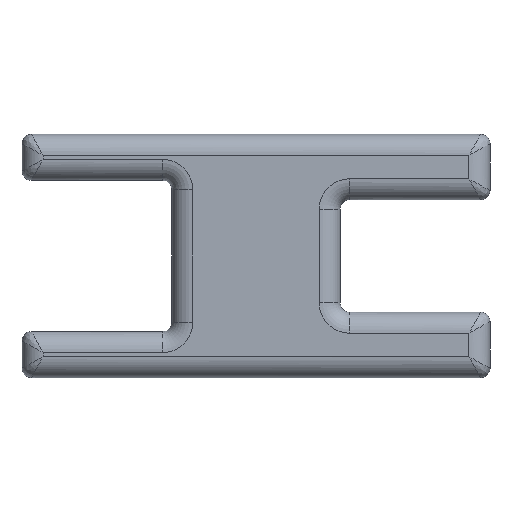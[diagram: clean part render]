
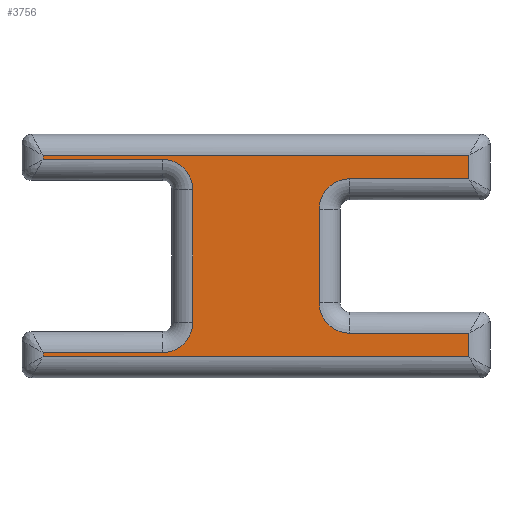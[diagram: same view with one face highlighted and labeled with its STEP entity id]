
A CAD part, front view. The second image highlights one B-rep face of the part: STEP entity #3756.
In plain terms, the highlighted planar face has unit normal (0, -1, 0).
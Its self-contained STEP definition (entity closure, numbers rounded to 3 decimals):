
#108=CIRCLE('',#3889,3.25);
#110=CIRCLE('',#3893,3.25);
#114=CIRCLE('',#3902,3.25);
#118=CIRCLE('',#3908,3.25);
#615=FACE_OUTER_BOUND('',#846,.T.);
#846=EDGE_LOOP('',(#3343,#3344,#3345,#3346,#3347,#3348,#3349,#3350,#3351,
#3352,#3353,#3354,#3355,#3356,#3357,#3358));
#1123=LINE('',#7339,#1422);
#1125=LINE('',#7348,#1424);
#1128=LINE('',#7360,#1427);
#1130=LINE('',#7366,#1429);
#1132=LINE('',#7369,#1431);
#1134=LINE('',#7372,#1433);
#1135=LINE('',#7375,#1434);
#1138=LINE('',#7390,#1437);
#1140=LINE('',#7399,#1439);
#1142=LINE('',#7402,#1441);
#1144=LINE('',#7405,#1443);
#1146=LINE('',#7408,#1445);
#1422=VECTOR('',#4404,10.);
#1424=VECTOR('',#4412,10.);
#1427=VECTOR('',#4427,10.);
#1429=VECTOR('',#4437,10.);
#1431=VECTOR('',#4441,10.);
#1433=VECTOR('',#4445,10.);
#1434=VECTOR('',#4448,10.);
#1437=VECTOR('',#4465,10.);
#1439=VECTOR('',#4477,10.);
#1441=VECTOR('',#4481,10.);
#1443=VECTOR('',#4485,10.);
#1445=VECTOR('',#4489,10.);
#1770=VERTEX_POINT('',#7082);
#1773=VERTEX_POINT('',#7118);
#1776=VERTEX_POINT('',#7154);
#1779=VERTEX_POINT('',#7190);
#1782=VERTEX_POINT('',#7226);
#1785=VERTEX_POINT('',#7262);
#1788=VERTEX_POINT('',#7298);
#1791=VERTEX_POINT('',#7334);
#1792=VERTEX_POINT('',#7338);
#1795=VERTEX_POINT('',#7345);
#1796=VERTEX_POINT('',#7347);
#1798=VERTEX_POINT('',#7353);
#1800=VERTEX_POINT('',#7374);
#1802=VERTEX_POINT('',#7380);
#1804=VERTEX_POINT('',#7386);
#1806=VERTEX_POINT('',#7392);
#2277=EDGE_CURVE('',#1770,#1792,#1123,.T.);
#2281=EDGE_CURVE('',#1795,#1796,#1125,.T.);
#2286=EDGE_CURVE('',#1796,#1798,#108,.T.);
#2288=EDGE_CURVE('',#1798,#1791,#1128,.T.);
#2290=EDGE_CURVE('',#1792,#1795,#110,.T.);
#2292=EDGE_CURVE('',#1791,#1788,#1130,.T.);
#2294=EDGE_CURVE('',#1788,#1785,#1132,.T.);
#2296=EDGE_CURVE('',#1785,#1782,#1134,.T.);
#2297=EDGE_CURVE('',#1782,#1800,#1135,.T.);
#2302=EDGE_CURVE('',#1800,#1802,#114,.T.);
#2305=EDGE_CURVE('',#1802,#1804,#1138,.T.);
#2308=EDGE_CURVE('',#1804,#1806,#118,.T.);
#2310=EDGE_CURVE('',#1806,#1779,#1140,.T.);
#2312=EDGE_CURVE('',#1779,#1776,#1142,.T.);
#2314=EDGE_CURVE('',#1776,#1773,#1144,.T.);
#2316=EDGE_CURVE('',#1773,#1770,#1146,.T.);
#3343=ORIENTED_EDGE('',*,*,#2281,.F.);
#3344=ORIENTED_EDGE('',*,*,#2290,.F.);
#3345=ORIENTED_EDGE('',*,*,#2277,.F.);
#3346=ORIENTED_EDGE('',*,*,#2316,.F.);
#3347=ORIENTED_EDGE('',*,*,#2314,.F.);
#3348=ORIENTED_EDGE('',*,*,#2312,.F.);
#3349=ORIENTED_EDGE('',*,*,#2310,.F.);
#3350=ORIENTED_EDGE('',*,*,#2308,.F.);
#3351=ORIENTED_EDGE('',*,*,#2305,.F.);
#3352=ORIENTED_EDGE('',*,*,#2302,.F.);
#3353=ORIENTED_EDGE('',*,*,#2297,.F.);
#3354=ORIENTED_EDGE('',*,*,#2296,.F.);
#3355=ORIENTED_EDGE('',*,*,#2294,.F.);
#3356=ORIENTED_EDGE('',*,*,#2292,.F.);
#3357=ORIENTED_EDGE('',*,*,#2288,.F.);
#3358=ORIENTED_EDGE('',*,*,#2286,.F.);
#3566=PLANE('',#3931);
#3756=ADVANCED_FACE('',(#615),#3566,.F.);
#3889=AXIS2_PLACEMENT_3D('',#7357,#4422,#4423);
#3893=AXIS2_PLACEMENT_3D('',#7363,#4432,#4433);
#3902=AXIS2_PLACEMENT_3D('',#7384,#4458,#4459);
#3908=AXIS2_PLACEMENT_3D('',#7396,#4472,#4473);
#3931=AXIS2_PLACEMENT_3D('',#7459,#4545,#4546);
#4404=DIRECTION('',(-1.,0.,0.));
#4412=DIRECTION('',(0.,0.,-1.));
#4422=DIRECTION('center_axis',(0.,-1.,0.));
#4423=DIRECTION('ref_axis',(-0.707,0.,-0.707));
#4427=DIRECTION('',(1.,0.,0.));
#4432=DIRECTION('center_axis',(0.,-1.,0.));
#4433=DIRECTION('ref_axis',(-0.707,0.,0.707));
#4437=DIRECTION('',(0.,0.,-1.));
#4441=DIRECTION('',(-1.,0.,0.));
#4445=DIRECTION('',(0.,0.,1.));
#4448=DIRECTION('',(1.,0.,0.));
#4458=DIRECTION('center_axis',(0.,-1.,0.));
#4459=DIRECTION('ref_axis',(0.707,0.,-0.707));
#4465=DIRECTION('',(0.,0.,1.));
#4472=DIRECTION('center_axis',(0.,-1.,0.));
#4473=DIRECTION('ref_axis',(0.707,0.,0.707));
#4477=DIRECTION('',(-1.,0.,0.));
#4481=DIRECTION('',(0.,0.,1.));
#4485=DIRECTION('',(1.,0.,0.));
#4489=DIRECTION('',(0.,0.,-1.));
#4545=DIRECTION('center_axis',(0.,1.,0.));
#4546=DIRECTION('ref_axis',(1.,0.,0.));
#7082=CARTESIAN_POINT('',(47.75,0.,-4.75));
#7118=CARTESIAN_POINT('',(47.75,0.,-2.25));
#7154=CARTESIAN_POINT('',(2.25,0.,-2.25));
#7190=CARTESIAN_POINT('',(2.25,0.,-2.675));
#7226=CARTESIAN_POINT('',(2.25,0.,-23.325));
#7262=CARTESIAN_POINT('',(2.25,0.,-23.75));
#7298=CARTESIAN_POINT('',(47.75,0.,-23.75));
#7334=CARTESIAN_POINT('',(47.75,0.,-21.25));
#7338=CARTESIAN_POINT('',(35.,0.,-4.75));
#7339=CARTESIAN_POINT('',(37.5,0.,-4.75));
#7345=CARTESIAN_POINT('',(31.75,0.,-8.));
#7347=CARTESIAN_POINT('',(31.75,0.,-18.));
#7348=CARTESIAN_POINT('',(31.75,0.,-10.));
#7353=CARTESIAN_POINT('',(35.,0.,-21.25));
#7357=CARTESIAN_POINT('Origin',(35.,0.,-18.));
#7360=CARTESIAN_POINT('',(29.5,0.,-21.25));
#7363=CARTESIAN_POINT('Origin',(35.,0.,-8.));
#7366=CARTESIAN_POINT('',(47.75,0.,-6.5));
#7369=CARTESIAN_POINT('',(37.5,0.,-23.75));
#7372=CARTESIAN_POINT('',(2.25,0.,-19.5));
#7374=CARTESIAN_POINT('',(15.,0.,-23.325));
#7375=CARTESIAN_POINT('',(12.5,0.,-23.325));
#7380=CARTESIAN_POINT('',(18.25,0.,-20.075));
#7384=CARTESIAN_POINT('Origin',(15.,0.,-20.075));
#7386=CARTESIAN_POINT('',(18.25,0.,-5.925));
#7390=CARTESIAN_POINT('',(18.25,0.,-16.75));
#7392=CARTESIAN_POINT('',(15.,0.,-2.675));
#7396=CARTESIAN_POINT('Origin',(15.,0.,-5.925));
#7399=CARTESIAN_POINT('',(20.5,0.,-2.675));
#7402=CARTESIAN_POINT('',(2.25,0.,-19.5));
#7405=CARTESIAN_POINT('',(12.5,0.,-2.25));
#7408=CARTESIAN_POINT('',(47.75,0.,-6.5));
#7459=CARTESIAN_POINT('Origin',(25.,0.,-13.));
